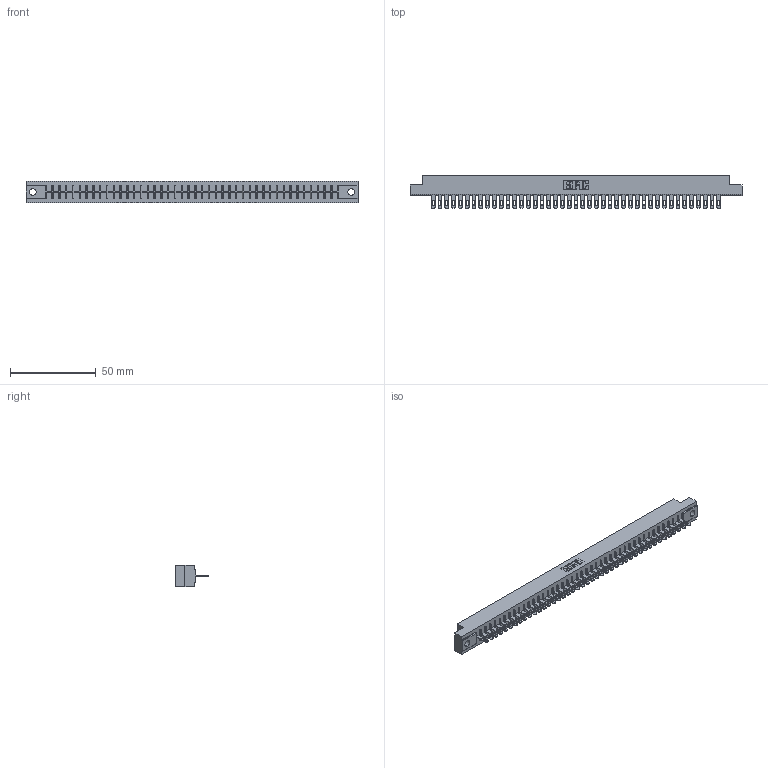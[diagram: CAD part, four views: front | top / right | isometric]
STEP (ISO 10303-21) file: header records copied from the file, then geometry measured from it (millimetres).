
FILE_DESCRIPTION (( 'STEP AP203' ), '1' );
FILE_NAME ('306-043-400-104.STEP', '2020-09-22T13:16:57', ( '' ), ( '' ), 'SwSTEP 2.0', 'SolidWorks 2020', '' );
FILE_SCHEMA (( 'CONFIG_CONTROL_DESIGN' ));
Length unit declared in the file: inch
Products named in the file (3): 306-043-400-104; 306 Part_.156 Dia; 306-290-001_100
Assembly tree (44 placements, depth 2):
  306-043-400-104
    306 Part_.156 Dia
    306-290-001_100  x43
Bounding box: 193.4 x 18.87 x 12.7 mm (x, y, z)
Volume: 21429.4 mm3; surface area: 22582.2 mm2
Topology: 44 solids, 44 shells, 3398 faces, 9597 edges, 6166 vertices
Faces by surface type: plane 2232, cylinder 994, sphere 172
Entity records: 40552 total; most frequent: CARTESIAN_POINT 6814, ORIENTED_EDGE 6754, DIRECTION 6711, EDGE_CURVE 3377, LINE 2649, VECTOR 2649, VERTEX_POINT 2134, AXIS2_PLACEMENT_3D 2031
